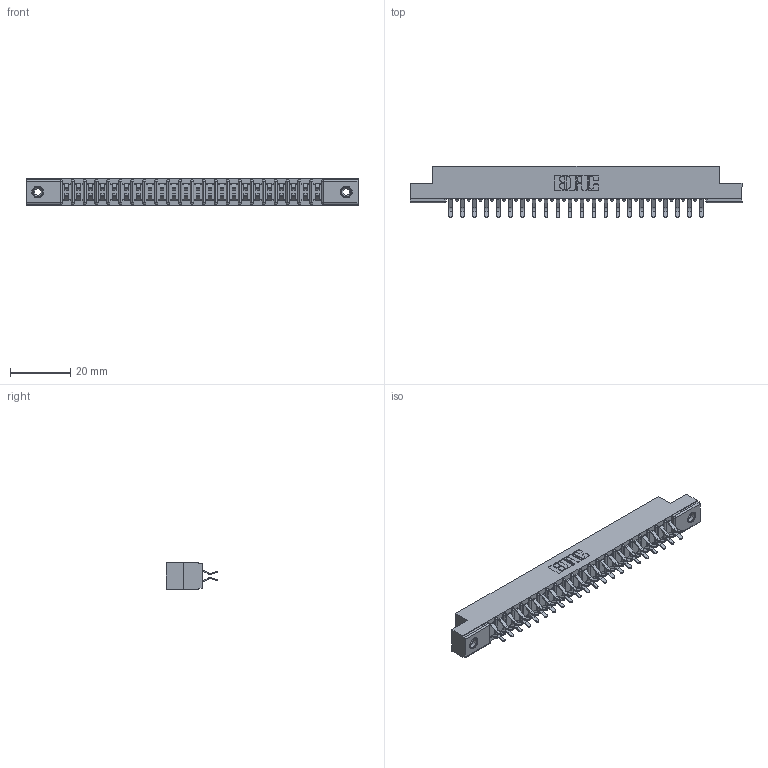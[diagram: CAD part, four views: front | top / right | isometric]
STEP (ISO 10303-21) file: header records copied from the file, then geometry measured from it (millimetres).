
FILE_DESCRIPTION (( 'STEP AP203' ), '1' );
FILE_NAME ('357-044-556-208.STEP', '2018-08-11T12:30:01', ( '' ), ( '' ), 'SwSTEP 2.0', 'SolidWorks 2016', '' );
FILE_SCHEMA (( 'CONFIG_CONTROL_DESIGN' ));
Length unit declared in the file: inch
Products named in the file (4): 307-290-001_556; 345-250-001_345-250-003-102; 357-044-556-208; 307 Part_.156 Dia Mounting Holes
Assembly tree (47 placements, depth 2):
  357-044-556-208
    307 Part_.156 Dia Mounting Holes
    307-290-001_556  x44
    345-250-001_345-250-003-102  x2
Bounding box: 110.19 x 16.97 x 8.71 mm (x, y, z)
Volume: 7192.8 mm3; surface area: 12681.9 mm2
Topology: 47 solids, 47 shells, 2401 faces, 6707 edges, 4342 vertices
Faces by surface type: plane 1554, cylinder 785, sphere 46, cone 12, torus 4
Entity records: 23319 total; most frequent: CARTESIAN_POINT 3805, ORIENTED_EDGE 3762, DIRECTION 3745, EDGE_CURVE 1881, LINE 1433, VECTOR 1433, VERTEX_POINT 1216, AXIS2_PLACEMENT_3D 1156
